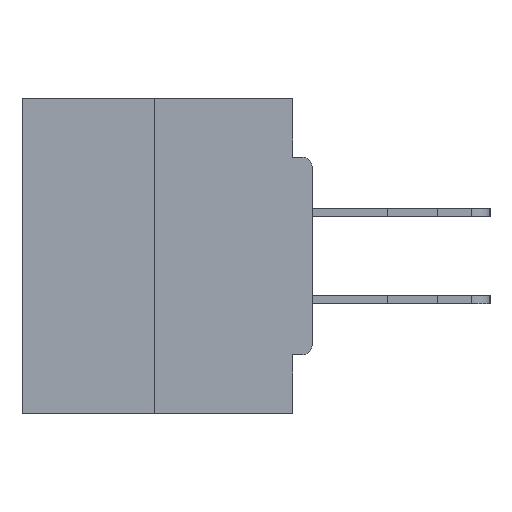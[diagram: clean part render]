
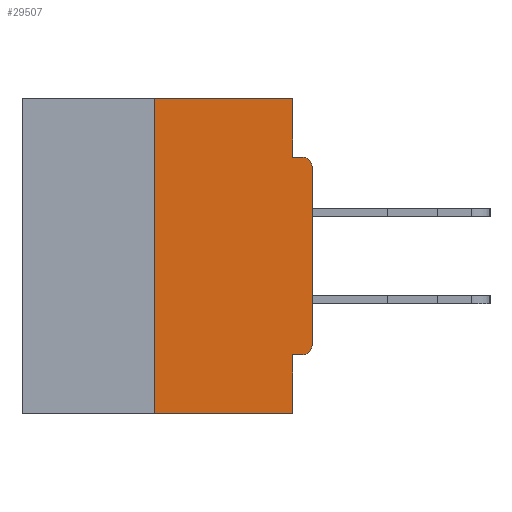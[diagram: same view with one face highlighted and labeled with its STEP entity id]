
A CAD part, left-side view. The second image highlights one B-rep face of the part: STEP entity #29507.
In plain terms, the highlighted planar face has unit normal (-1, 0, 0).
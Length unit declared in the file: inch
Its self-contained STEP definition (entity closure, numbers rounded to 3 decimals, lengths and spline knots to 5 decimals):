
#1370 = DIRECTION ( 'NONE',  ( 0., 0., -1. ) ) ;
#1491 = CARTESIAN_POINT ( 'NONE',  ( 0., 0.015, -0.3915 ) ) ;
#2901 = VERTEX_POINT ( 'NONE', #18330 ) ;
#3024 = VERTEX_POINT ( 'NONE', #24362 ) ;
#3046 = EDGE_CURVE ( 'NONE', #3024, #11756, #4478, .T. ) ;
#3370 = CARTESIAN_POINT ( 'NONE',  ( 0., 0., -0.1085 ) ) ;
#3543 = CIRCLE ( 'NONE', #14380, 0.015 ) ;
#4089 = DIRECTION ( 'NONE',  ( -1., 0., 0. ) ) ;
#4326 = ORIENTED_EDGE ( 'NONE', *, *, #14585, .F. ) ;
#4478 = LINE ( 'NONE', #24243, #9362 ) ;
#4523 = PLANE ( 'NONE',  #27414 ) ;
#5462 = ORIENTED_EDGE ( 'NONE', *, *, #3046, .F. ) ;
#5678 = VECTOR ( 'NONE', #29609, 39.37008 ) ;
#6991 = CARTESIAN_POINT ( 'NONE',  ( 0., 0.031, 0. ) ) ;
#7083 = CIRCLE ( 'NONE', #25997, 0.015 ) ;
#7633 = EDGE_CURVE ( 'NONE', #2901, #31349, #34447, .T. ) ;
#8294 = EDGE_CURVE ( 'NONE', #3024, #17580, #3543, .T. ) ;
#8622 = VECTOR ( 'NONE', #14507, 39.37008 ) ;
#9362 = VECTOR ( 'NONE', #27266, 39.37008 ) ;
#9376 = VECTOR ( 'NONE', #20647, 39.37008 ) ;
#9634 = LINE ( 'NONE', #9954, #5678 ) ;
#9661 = CARTESIAN_POINT ( 'NONE',  ( 0., 0.031, -0.5 ) ) ;
#9954 = CARTESIAN_POINT ( 'NONE',  ( 0., 0.031, 0. ) ) ;
#9977 = VERTEX_POINT ( 'NONE', #25341 ) ;
#11160 = EDGE_LOOP ( 'NONE', ( #31436, #15105, #17884, #4326, #5462, #27247, #24966, #15751, #31779, #27225 ) ) ;
#11756 = VERTEX_POINT ( 'NONE', #20549 ) ;
#11893 = VERTEX_POINT ( 'NONE', #6991 ) ;
#12848 = DIRECTION ( 'NONE',  ( -1., 0., 0. ) ) ;
#13214 = EDGE_CURVE ( 'NONE', #28435, #21584, #15148, .T. ) ;
#13607 = CARTESIAN_POINT ( 'NONE',  ( 0., 0., -0.3915 ) ) ;
#14380 = AXIS2_PLACEMENT_3D ( 'NONE', #1491, #12848, #30398 ) ;
#14507 = DIRECTION ( 'NONE',  ( 0., -1., 0. ) ) ;
#14585 = EDGE_CURVE ( 'NONE', #11756, #9977, #27587, .T. ) ;
#14646 = VECTOR ( 'NONE', #29551, 39.37008 ) ;
#15105 = ORIENTED_EDGE ( 'NONE', *, *, #7633, .F. ) ;
#15148 = LINE ( 'NONE', #28960, #9376 ) ;
#15289 = EDGE_CURVE ( 'NONE', #33870, #21584, #7083, .T. ) ;
#15751 = ORIENTED_EDGE ( 'NONE', *, *, #15289, .T. ) ;
#16569 = CARTESIAN_POINT ( 'NONE',  ( 0., 0.46, 0. ) ) ;
#16990 = EDGE_CURVE ( 'NONE', #17580, #33870, #21638, .T. ) ;
#17580 = VERTEX_POINT ( 'NONE', #13607 ) ;
#17884 = ORIENTED_EDGE ( 'NONE', *, *, #30540, .T. ) ;
#18330 = CARTESIAN_POINT ( 'NONE',  ( 0., 0.25, -0.5 ) ) ;
#20549 = CARTESIAN_POINT ( 'NONE',  ( 0., 0.031, -0.4065 ) ) ;
#20647 = DIRECTION ( 'NONE',  ( 0., -1., 0. ) ) ;
#21584 = VERTEX_POINT ( 'NONE', #27406 ) ;
#21638 = LINE ( 'NONE', #30228, #23867 ) ;
#23867 = VECTOR ( 'NONE', #33133, 39.37008 ) ;
#24243 = CARTESIAN_POINT ( 'NONE',  ( 0., 0., -0.4065 ) ) ;
#24331 = CARTESIAN_POINT ( 'NONE',  ( 0., 0.25, 0. ) ) ;
#24362 = CARTESIAN_POINT ( 'NONE',  ( 0., 0.015, -0.4065 ) ) ;
#24939 = CARTESIAN_POINT ( 'NONE',  ( 0., 0.031, -0.0935 ) ) ;
#24966 = ORIENTED_EDGE ( 'NONE', *, *, #16990, .T. ) ;
#25317 = CARTESIAN_POINT ( 'NONE',  ( 0., 0.46, 0. ) ) ;
#25341 = CARTESIAN_POINT ( 'NONE',  ( 0., 0.031, -0.5 ) ) ;
#25753 = CARTESIAN_POINT ( 'NONE',  ( 0., 0.46, -0.5 ) ) ;
#25997 = AXIS2_PLACEMENT_3D ( 'NONE', #34455, #4089, #1370 ) ;
#26223 = EDGE_CURVE ( 'NONE', #11893, #28435, #9634, .T. ) ;
#26412 = FACE_OUTER_BOUND ( 'NONE', #11160, .T. ) ;
#27225 = ORIENTED_EDGE ( 'NONE', *, *, #26223, .F. ) ;
#27247 = ORIENTED_EDGE ( 'NONE', *, *, #8294, .T. ) ;
#27266 = DIRECTION ( 'NONE',  ( 0., 1., 0. ) ) ;
#27345 = DIRECTION ( 'NONE',  ( 0., 0., 1. ) ) ;
#27406 = CARTESIAN_POINT ( 'NONE',  ( 0., 0.015, -0.0935 ) ) ;
#27414 = AXIS2_PLACEMENT_3D ( 'NONE', #16569, #36372, #31113 ) ;
#27587 = LINE ( 'NONE', #9661, #14646 ) ;
#28207 = VECTOR ( 'NONE', #27345, 39.37008 ) ;
#28435 = VERTEX_POINT ( 'NONE', #24939 ) ;
#28595 = LINE ( 'NONE', #25753, #33480 ) ;
#28605 = DIRECTION ( 'NONE',  ( 0., -1., 0. ) ) ;
#28960 = CARTESIAN_POINT ( 'NONE',  ( 0., 0., -0.0935 ) ) ;
#29507 = ADVANCED_FACE ( 'NONE', ( #26412 ), #4523, .F. ) ;
#29551 = DIRECTION ( 'NONE',  ( 0., 0., -1. ) ) ;
#29609 = DIRECTION ( 'NONE',  ( 0., 0., -1. ) ) ;
#29771 = EDGE_CURVE ( 'NONE', #31349, #11893, #34448, .T. ) ;
#30228 = CARTESIAN_POINT ( 'NONE',  ( 0., 0., 0. ) ) ;
#30398 = DIRECTION ( 'NONE',  ( 0., 0., -1. ) ) ;
#30540 = EDGE_CURVE ( 'NONE', #2901, #9977, #28595, .T. ) ;
#31113 = DIRECTION ( 'NONE',  ( 0., 0., -1. ) ) ;
#31349 = VERTEX_POINT ( 'NONE', #34230 ) ;
#31436 = ORIENTED_EDGE ( 'NONE', *, *, #29771, .F. ) ;
#31779 = ORIENTED_EDGE ( 'NONE', *, *, #13214, .F. ) ;
#33133 = DIRECTION ( 'NONE',  ( 0., 0., 1. ) ) ;
#33480 = VECTOR ( 'NONE', #28605, 39.37008 ) ;
#33870 = VERTEX_POINT ( 'NONE', #3370 ) ;
#34230 = CARTESIAN_POINT ( 'NONE',  ( 0., 0.25, 0. ) ) ;
#34447 = LINE ( 'NONE', #24331, #28207 ) ;
#34448 = LINE ( 'NONE', #25317, #8622 ) ;
#34455 = CARTESIAN_POINT ( 'NONE',  ( 0., 0.015, -0.1085 ) ) ;
#36372 = DIRECTION ( 'NONE',  ( 1., 0., 0. ) ) ;
